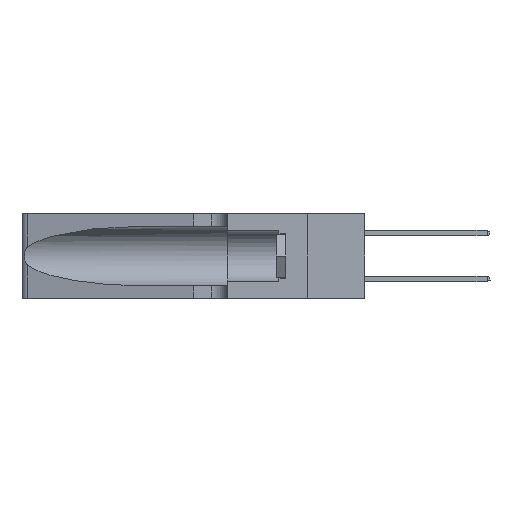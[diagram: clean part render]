
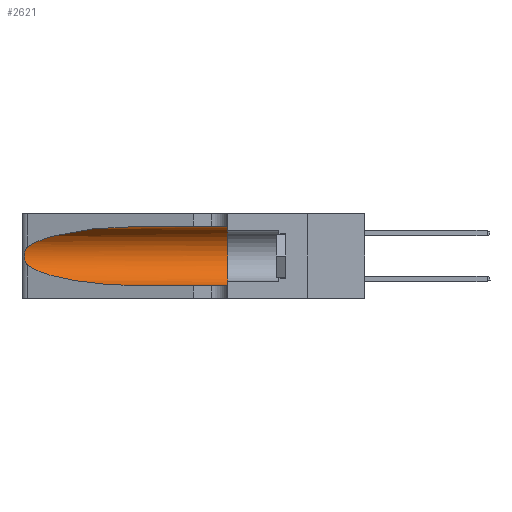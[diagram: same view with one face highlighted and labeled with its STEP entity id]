
A CAD part, left-side view. The second image highlights one B-rep face of the part: STEP entity #2621.
In plain terms, the highlighted cylindrical face has radius 3.308 mm (diameter 6.617 mm), a partial arc.
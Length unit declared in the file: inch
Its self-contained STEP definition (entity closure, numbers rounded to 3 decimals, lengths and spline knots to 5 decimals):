
#78 = VERTEX_POINT ( 'NONE', #14623 ) ;
#734 = CARTESIAN_POINT ( 'NONE',  ( 0.1305, 0.35, 0.185 ) ) ;
#960 = LINE ( 'NONE', #8336, #11260 ) ;
#1259 = CARTESIAN_POINT ( 'NONE',  ( 0.25639, 1.23186, 0.15144 ) ) ;
#1503 = B_SPLINE_CURVE_WITH_KNOTS ( 'NONE', 3,
 ( #14203, #3425, #5628, #20753, #7802, #22898, #9995, #25007, #12192, #27104, #14397, #1259, #16568, #3521 ),
 .UNSPECIFIED., .F., .F.,
 ( 4, 2, 2, 2, 2, 2, 4 ),
 ( 0., 0.00027, 0.00053, 0.00107, 0.0016, 0.00187, 0.00214 ),
 .UNSPECIFIED. ) ;
#2621 = ADVANCED_FACE ( 'NONE', ( #6726 ), #22618, .F. ) ;
#2861 = CARTESIAN_POINT ( 'NONE',  ( 0.1305, 1.61858, 0.185 ) ) ;
#3015 = DIRECTION ( 'NONE',  ( 0., 0., 1. ) ) ;
#3425 = CARTESIAN_POINT ( 'NONE',  ( 0.25555, 1.22994, 0.2215 ) ) ;
#3521 = CARTESIAN_POINT ( 'NONE',  ( 0.25487, 1.22718, 0.14631 ) ) ;
#3829 = LINE ( 'NONE', #21343, #19749 ) ;
#4923 = CARTESIAN_POINT ( 'NONE',  ( 0.1305, 0.72297, 0.05475 ) ) ;
#5198 = ORIENTED_EDGE ( 'NONE', *, *, #17558, .T. ) ;
#5628 = CARTESIAN_POINT ( 'NONE',  ( 0.25639, 1.23184, 0.21858 ) ) ;
#6726 = FACE_OUTER_BOUND ( 'NONE', #13153, .T. ) ;
#7285 = EDGE_CURVE ( 'NONE', #25294, #27622, #960, .T. ) ;
#7802 = CARTESIAN_POINT ( 'NONE',  ( 0.25854, 1.2359, 0.20912 ) ) ;
#7838 = EDGE_CURVE ( 'NONE', #18125, #18019, #3829, .T. ) ;
#7863 = CARTESIAN_POINT ( 'NONE',  ( 0.1305, 0.35, 0.31525 ) ) ;
#8336 = CARTESIAN_POINT ( 'NONE',  ( 0.1305, 1.61858, 0.05475 ) ) ;
#9810 = ORIENTED_EDGE ( 'NONE', *, *, #10987, .T. ) ;
#9995 = CARTESIAN_POINT ( 'NONE',  ( 0.26075, 1.23896, 0.19203 ) ) ;
#10432 = CARTESIAN_POINT ( 'NONE',  ( 0.1305, 0.72297, 0.31525 ) ) ;
#10595 = CIRCLE ( 'NONE', #16754, 0.13025 ) ;
#10692 = AXIS2_PLACEMENT_3D ( 'NONE', #2861, #13828, #11643 ) ;
#10776 = CARTESIAN_POINT ( 'NONE',  ( 0.25487, 1.22718, 0.14631 ) ) ;
#10880 = CARTESIAN_POINT ( 'NONE',  ( 0.18966, 0.96281, 0.31525 ) ) ;
#10987 = EDGE_CURVE ( 'NONE', #18125, #78, #26598, .T. ) ;
#11260 = VECTOR ( 'NONE', #14834, 39.37008 ) ;
#11643 = DIRECTION ( 'NONE',  ( 0., 0., -1. ) ) ;
#11699 =( BOUNDED_CURVE ( )  B_SPLINE_CURVE ( 3, ( #15035, #27736, #12822, #17219 ),
 .UNSPECIFIED., .F., .F. ) 
 B_SPLINE_CURVE_WITH_KNOTS ( ( 4, 4 ),
 ( 3.44316, 4.71239 ),
 .UNSPECIFIED. ) 
 CURVE ( )  GEOMETRIC_REPRESENTATION_ITEM ( )  RATIONAL_B_SPLINE_CURVE ( ( 1., 0.87, 0.87, 1. ) ) 
 REPRESENTATION_ITEM ( '' )  );
#12192 = CARTESIAN_POINT ( 'NONE',  ( 0.26017, 1.23833, 0.17102 ) ) ;
#12822 = CARTESIAN_POINT ( 'NONE',  ( 0.18966, 0.96281, 0.05475 ) ) ;
#13041 = CARTESIAN_POINT ( 'NONE',  ( 0.1305, 0.35, 0.05475 ) ) ;
#13153 = EDGE_LOOP ( 'NONE', ( #9810, #15395, #5198, #20088, #16440, #20055 ) ) ;
#13828 = DIRECTION ( 'NONE',  ( 0., -1., 0. ) ) ;
#14203 = CARTESIAN_POINT ( 'NONE',  ( 0.25487, 1.22718, 0.22369 ) ) ;
#14397 = CARTESIAN_POINT ( 'NONE',  ( 0.25789, 1.23486, 0.15765 ) ) ;
#14623 = CARTESIAN_POINT ( 'NONE',  ( 0.25487, 1.22718, 0.22369 ) ) ;
#14834 = DIRECTION ( 'NONE',  ( 0., -1., 0. ) ) ;
#15035 = CARTESIAN_POINT ( 'NONE',  ( 0.25487, 1.22718, 0.14631 ) ) ;
#15264 = CARTESIAN_POINT ( 'NONE',  ( 0.25487, 1.22718, 0.22369 ) ) ;
#15395 = ORIENTED_EDGE ( 'NONE', *, *, #20089, .T. ) ;
#15759 = EDGE_CURVE ( 'NONE', #18019, #27622, #10595, .T. ) ;
#16068 = DIRECTION ( 'NONE',  ( 0., 1., 0. ) ) ;
#16440 = ORIENTED_EDGE ( 'NONE', *, *, #15759, .F. ) ;
#16568 = CARTESIAN_POINT ( 'NONE',  ( 0.25555, 1.22993, 0.14849 ) ) ;
#16754 = AXIS2_PLACEMENT_3D ( 'NONE', #734, #16068, #3015 ) ;
#17219 = CARTESIAN_POINT ( 'NONE',  ( 0.1305, 0.72297, 0.05475 ) ) ;
#17353 = CARTESIAN_POINT ( 'NONE',  ( 0.1305, 0.72297, 0.31525 ) ) ;
#17558 = EDGE_CURVE ( 'NONE', #25772, #25294, #11699, .T. ) ;
#18019 = VERTEX_POINT ( 'NONE', #7863 ) ;
#18125 = VERTEX_POINT ( 'NONE', #10432 ) ;
#19749 = VECTOR ( 'NONE', #23481, 39.37008 ) ;
#20055 = ORIENTED_EDGE ( 'NONE', *, *, #7838, .F. ) ;
#20088 = ORIENTED_EDGE ( 'NONE', *, *, #7285, .T. ) ;
#20089 = EDGE_CURVE ( 'NONE', #78, #25772, #1503, .T. ) ;
#20753 = CARTESIAN_POINT ( 'NONE',  ( 0.25787, 1.23484, 0.2124 ) ) ;
#21343 = CARTESIAN_POINT ( 'NONE',  ( 0.1305, 1.61858, 0.31525 ) ) ;
#22618 = CYLINDRICAL_SURFACE ( 'NONE', #10692, 0.13025 ) ;
#22898 = CARTESIAN_POINT ( 'NONE',  ( 0.26018, 1.23835, 0.19895 ) ) ;
#23481 = DIRECTION ( 'NONE',  ( 0., -1., 0. ) ) ;
#25007 = CARTESIAN_POINT ( 'NONE',  ( 0.26075, 1.23896, 0.178 ) ) ;
#25294 = VERTEX_POINT ( 'NONE', #4923 ) ;
#25772 = VERTEX_POINT ( 'NONE', #10776 ) ;
#26598 =( BOUNDED_CURVE ( )  B_SPLINE_CURVE ( 3, ( #17353, #10880, #27952, #15264 ),
 .UNSPECIFIED., .F., .F. ) 
 B_SPLINE_CURVE_WITH_KNOTS ( ( 4, 4 ),
 ( 1.5708, 2.84003 ),
 .UNSPECIFIED. ) 
 CURVE ( )  GEOMETRIC_REPRESENTATION_ITEM ( )  RATIONAL_B_SPLINE_CURVE ( ( 1., 0.87, 0.87, 1. ) ) 
 REPRESENTATION_ITEM ( '' )  );
#27104 = CARTESIAN_POINT ( 'NONE',  ( 0.25856, 1.23593, 0.16098 ) ) ;
#27622 = VERTEX_POINT ( 'NONE', #13041 ) ;
#27736 = CARTESIAN_POINT ( 'NONE',  ( 0.2373, 1.15595, 0.08982 ) ) ;
#27952 = CARTESIAN_POINT ( 'NONE',  ( 0.2373, 1.15595, 0.28018 ) ) ;
